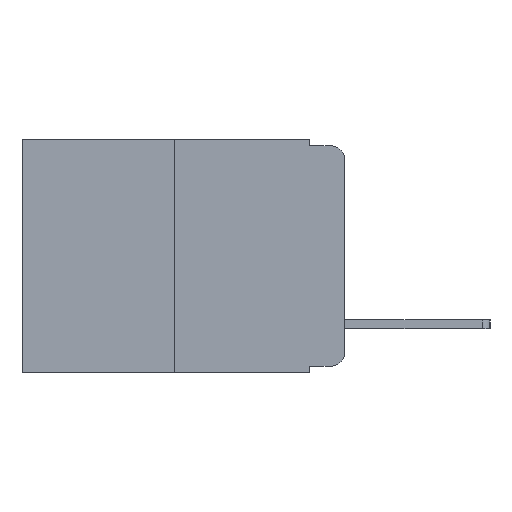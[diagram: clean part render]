
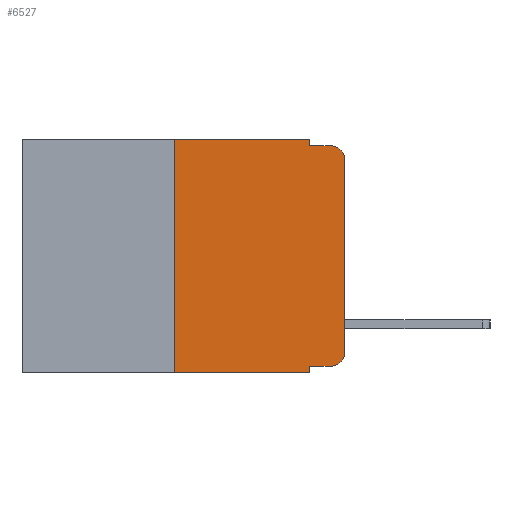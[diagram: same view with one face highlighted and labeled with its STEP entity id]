
A CAD part, left-side view. The second image highlights one B-rep face of the part: STEP entity #6527.
In plain terms, the highlighted planar face has unit normal (-1, 0, 0).
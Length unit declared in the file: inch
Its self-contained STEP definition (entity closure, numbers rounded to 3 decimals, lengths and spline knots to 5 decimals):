
#34 = CARTESIAN_POINT ( 'NONE',  ( 0., 0.051, -0.01 ) ) ;
#161 = EDGE_LOOP ( 'NONE', ( #10291, #4688, #7802, #5055, #8155, #10917, #13513, #5443, #8548, #5806 ) ) ;
#883 = DIRECTION ( 'NONE',  ( 0., -1., 0. ) ) ;
#940 = VERTEX_POINT ( 'NONE', #12838 ) ;
#1050 = VERTEX_POINT ( 'NONE', #6168 ) ;
#1132 = LINE ( 'NONE', #12620, #9585 ) ;
#1441 = CIRCLE ( 'NONE', #11059, 0.02 ) ;
#1725 = VERTEX_POINT ( 'NONE', #3414 ) ;
#1749 = VERTEX_POINT ( 'NONE', #3453 ) ;
#1807 = VECTOR ( 'NONE', #9703, 39.37008 ) ;
#1903 = VECTOR ( 'NONE', #3637, 39.37008 ) ;
#2318 = LINE ( 'NONE', #3948, #10723 ) ;
#2371 = LINE ( 'NONE', #7028, #1903 ) ;
#2406 = CARTESIAN_POINT ( 'NONE',  ( 0., 0.051, 0. ) ) ;
#2931 = EDGE_CURVE ( 'NONE', #10349, #1749, #6089, .T. ) ;
#3223 = VERTEX_POINT ( 'NONE', #10503 ) ;
#3359 = VERTEX_POINT ( 'NONE', #5497 ) ;
#3414 = CARTESIAN_POINT ( 'NONE',  ( 0., 0., -0.03 ) ) ;
#3453 = CARTESIAN_POINT ( 'NONE',  ( 0., 0.051, 0. ) ) ;
#3454 = DIRECTION ( 'NONE',  ( 0., 0., -1. ) ) ;
#3637 = DIRECTION ( 'NONE',  ( 0., 0., 1. ) ) ;
#3948 = CARTESIAN_POINT ( 'NONE',  ( 0., 0.051, -0.333 ) ) ;
#4003 = DIRECTION ( 'NONE',  ( 0., 0., -1. ) ) ;
#4223 = CARTESIAN_POINT ( 'NONE',  ( 0., 0.473, 0. ) ) ;
#4270 = DIRECTION ( 'NONE',  ( -1., 0., 0. ) ) ;
#4290 = CARTESIAN_POINT ( 'NONE',  ( 0., 0.02, -0.313 ) ) ;
#4362 = VERTEX_POINT ( 'NONE', #11732 ) ;
#4562 = AXIS2_PLACEMENT_3D ( 'NONE', #8423, #11494, #4950 ) ;
#4613 = FACE_OUTER_BOUND ( 'NONE', #161, .T. ) ;
#4688 = ORIENTED_EDGE ( 'NONE', *, *, #9980, .T. ) ;
#4698 = EDGE_CURVE ( 'NONE', #940, #7051, #1441, .T. ) ;
#4900 = EDGE_CURVE ( 'NONE', #3359, #4362, #12834, .T. ) ;
#4950 = DIRECTION ( 'NONE',  ( 0., 0., -1. ) ) ;
#5055 = ORIENTED_EDGE ( 'NONE', *, *, #8611, .F. ) ;
#5395 = CIRCLE ( 'NONE', #13768, 0.02 ) ;
#5442 = VECTOR ( 'NONE', #12158, 39.37008 ) ;
#5443 = ORIENTED_EDGE ( 'NONE', *, *, #6284, .F. ) ;
#5497 = CARTESIAN_POINT ( 'NONE',  ( 0., 0.25, -0.343 ) ) ;
#5502 = EDGE_CURVE ( 'NONE', #5560, #940, #2318, .T. ) ;
#5511 = DIRECTION ( 'NONE',  ( 0., -1., 0. ) ) ;
#5560 = VERTEX_POINT ( 'NONE', #8649 ) ;
#5598 = CARTESIAN_POINT ( 'NONE',  ( 0., 0.02, -0.03 ) ) ;
#5806 = ORIENTED_EDGE ( 'NONE', *, *, #4698, .T. ) ;
#6089 = LINE ( 'NONE', #4223, #13759 ) ;
#6168 = CARTESIAN_POINT ( 'NONE',  ( 0., 0.02, -0.01 ) ) ;
#6284 = EDGE_CURVE ( 'NONE', #5560, #4362, #1132, .T. ) ;
#6328 = VECTOR ( 'NONE', #5511, 39.37008 ) ;
#6527 = ADVANCED_FACE ( 'NONE', ( #4613 ), #7255, .F. ) ;
#6766 = DIRECTION ( 'NONE',  ( 0., 0., -1. ) ) ;
#7028 = CARTESIAN_POINT ( 'NONE',  ( 0., 0.25, 0. ) ) ;
#7051 = VERTEX_POINT ( 'NONE', #8914 ) ;
#7255 = PLANE ( 'NONE',  #4562 ) ;
#7538 = CARTESIAN_POINT ( 'NONE',  ( 0., 0.473, -0.343 ) ) ;
#7636 = DIRECTION ( 'NONE',  ( 0., -1., 0. ) ) ;
#7802 = ORIENTED_EDGE ( 'NONE', *, *, #9297, .F. ) ;
#7837 = EDGE_CURVE ( 'NONE', #3359, #10349, #2371, .T. ) ;
#8155 = ORIENTED_EDGE ( 'NONE', *, *, #2931, .F. ) ;
#8423 = CARTESIAN_POINT ( 'NONE',  ( 0., 0.473, 0. ) ) ;
#8434 = CARTESIAN_POINT ( 'NONE',  ( 0., 0.25, 0. ) ) ;
#8504 = DIRECTION ( 'NONE',  ( 0., -1., 0. ) ) ;
#8529 = LINE ( 'NONE', #2406, #5442 ) ;
#8548 = ORIENTED_EDGE ( 'NONE', *, *, #5502, .T. ) ;
#8611 = EDGE_CURVE ( 'NONE', #1749, #3223, #8529, .T. ) ;
#8649 = CARTESIAN_POINT ( 'NONE',  ( 0., 0.051, -0.333 ) ) ;
#8914 = CARTESIAN_POINT ( 'NONE',  ( 0., 0., -0.313 ) ) ;
#9297 = EDGE_CURVE ( 'NONE', #3223, #1050, #12316, .T. ) ;
#9585 = VECTOR ( 'NONE', #4003, 39.37008 ) ;
#9703 = DIRECTION ( 'NONE',  ( 0., 0., 1. ) ) ;
#9980 = EDGE_CURVE ( 'NONE', #1725, #1050, #5395, .T. ) ;
#10291 = ORIENTED_EDGE ( 'NONE', *, *, #10653, .T. ) ;
#10349 = VERTEX_POINT ( 'NONE', #8434 ) ;
#10496 = VECTOR ( 'NONE', #883, 39.37008 ) ;
#10503 = CARTESIAN_POINT ( 'NONE',  ( 0., 0.051, -0.01 ) ) ;
#10541 = LINE ( 'NONE', #11859, #1807 ) ;
#10653 = EDGE_CURVE ( 'NONE', #7051, #1725, #10541, .T. ) ;
#10723 = VECTOR ( 'NONE', #8504, 39.37008 ) ;
#10917 = ORIENTED_EDGE ( 'NONE', *, *, #7837, .F. ) ;
#11059 = AXIS2_PLACEMENT_3D ( 'NONE', #4290, #4270, #3454 ) ;
#11494 = DIRECTION ( 'NONE',  ( 1., 0., 0. ) ) ;
#11732 = CARTESIAN_POINT ( 'NONE',  ( 0., 0.051, -0.343 ) ) ;
#11859 = CARTESIAN_POINT ( 'NONE',  ( 0., 0., 0. ) ) ;
#12158 = DIRECTION ( 'NONE',  ( 0., 0., -1. ) ) ;
#12316 = LINE ( 'NONE', #34, #6328 ) ;
#12620 = CARTESIAN_POINT ( 'NONE',  ( 0., 0.051, 0. ) ) ;
#12834 = LINE ( 'NONE', #7538, #10496 ) ;
#12838 = CARTESIAN_POINT ( 'NONE',  ( 0., 0.02, -0.333 ) ) ;
#13017 = DIRECTION ( 'NONE',  ( -1., 0., 0. ) ) ;
#13513 = ORIENTED_EDGE ( 'NONE', *, *, #4900, .T. ) ;
#13759 = VECTOR ( 'NONE', #7636, 39.37008 ) ;
#13768 = AXIS2_PLACEMENT_3D ( 'NONE', #5598, #13017, #6766 ) ;
